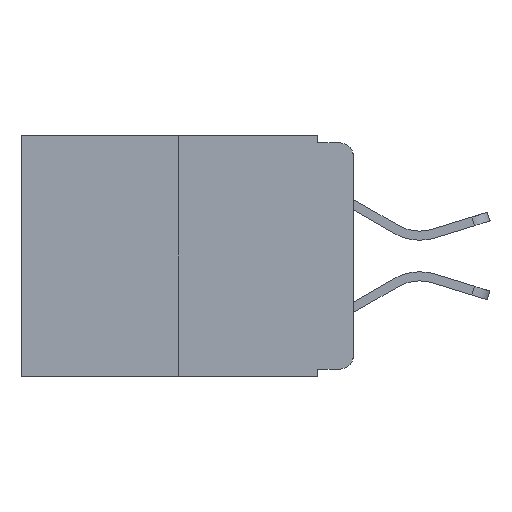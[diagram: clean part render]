
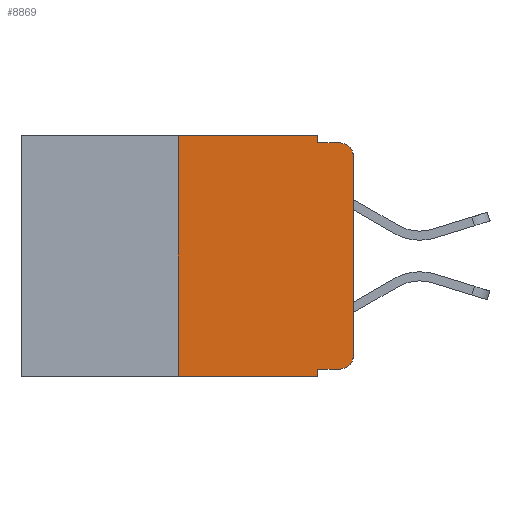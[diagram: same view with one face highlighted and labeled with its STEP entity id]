
A CAD part, left-side view. The second image highlights one B-rep face of the part: STEP entity #8869.
In plain terms, the highlighted planar face has unit normal (-1, 0, 0).
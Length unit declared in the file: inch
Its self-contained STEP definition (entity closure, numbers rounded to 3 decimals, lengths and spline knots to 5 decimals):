
#67 = ORIENTED_EDGE ( 'NONE', *, *, #6273, .F. ) ;
#86 = ORIENTED_EDGE ( 'NONE', *, *, #17245, .T. ) ;
#138 = VERTEX_POINT ( 'NONE', #15224 ) ;
#441 = CARTESIAN_POINT ( 'NONE',  ( 0., 0., -0.03 ) ) ;
#612 = EDGE_CURVE ( 'NONE', #138, #10915, #4521, .T. ) ;
#1225 = DIRECTION ( 'NONE',  ( 0., -1., 0. ) ) ;
#1445 = CARTESIAN_POINT ( 'NONE',  ( 0., 0.25, 0. ) ) ;
#1669 = DIRECTION ( 'NONE',  ( 0., -1., 0. ) ) ;
#1747 = EDGE_CURVE ( 'NONE', #2428, #138, #6983, .T. ) ;
#1871 = VECTOR ( 'NONE', #5521, 39.37008 ) ;
#2053 = DIRECTION ( 'NONE',  ( 0., 0., 1. ) ) ;
#2428 = VERTEX_POINT ( 'NONE', #8044 ) ;
#2484 = CARTESIAN_POINT ( 'NONE',  ( 0., 0.25, -0.343 ) ) ;
#2656 = CARTESIAN_POINT ( 'NONE',  ( 0., 0.473, 0. ) ) ;
#2791 = CARTESIAN_POINT ( 'NONE',  ( 0., 0.051, -0.333 ) ) ;
#2795 = EDGE_CURVE ( 'NONE', #9002, #14199, #11804, .T. ) ;
#3667 = LINE ( 'NONE', #18136, #10806 ) ;
#3687 = ORIENTED_EDGE ( 'NONE', *, *, #612, .T. ) ;
#3758 = VECTOR ( 'NONE', #16440, 39.37008 ) ;
#4008 = AXIS2_PLACEMENT_3D ( 'NONE', #2656, #12648, #4095 ) ;
#4095 = DIRECTION ( 'NONE',  ( 0., 0., -1. ) ) ;
#4148 = ORIENTED_EDGE ( 'NONE', *, *, #7474, .F. ) ;
#4521 = LINE ( 'NONE', #5185, #7886 ) ;
#5185 = CARTESIAN_POINT ( 'NONE',  ( 0., 0., 0. ) ) ;
#5221 = EDGE_CURVE ( 'NONE', #10643, #11042, #16909, .T. ) ;
#5313 = CARTESIAN_POINT ( 'NONE',  ( 0., 0.051, 0. ) ) ;
#5521 = DIRECTION ( 'NONE',  ( 0., -1., 0. ) ) ;
#5792 = LINE ( 'NONE', #8795, #12901 ) ;
#5870 = CARTESIAN_POINT ( 'NONE',  ( 0., 0.473, -0.343 ) ) ;
#6273 = EDGE_CURVE ( 'NONE', #16068, #11042, #18173, .T. ) ;
#6460 = CARTESIAN_POINT ( 'NONE',  ( 0., 0.02, -0.313 ) ) ;
#6477 = DIRECTION ( 'NONE',  ( -1., 0., 0. ) ) ;
#6510 = CARTESIAN_POINT ( 'NONE',  ( 0., 0.051, -0.343 ) ) ;
#6549 = DIRECTION ( 'NONE',  ( -1., 0., 0. ) ) ;
#6592 = DIRECTION ( 'NONE',  ( 0., 0., -1. ) ) ;
#6983 = CIRCLE ( 'NONE', #7169, 0.02 ) ;
#7169 = AXIS2_PLACEMENT_3D ( 'NONE', #6460, #6549, #6592 ) ;
#7174 = VECTOR ( 'NONE', #2053, 39.37008 ) ;
#7474 = EDGE_CURVE ( 'NONE', #10643, #9002, #14667, .T. ) ;
#7886 = VECTOR ( 'NONE', #10283, 39.37008 ) ;
#8044 = CARTESIAN_POINT ( 'NONE',  ( 0., 0.02, -0.333 ) ) ;
#8179 = CIRCLE ( 'NONE', #13635, 0.02 ) ;
#8515 = CARTESIAN_POINT ( 'NONE',  ( 0., 0.02, -0.01 ) ) ;
#8618 = ORIENTED_EDGE ( 'NONE', *, *, #2795, .F. ) ;
#8795 = CARTESIAN_POINT ( 'NONE',  ( 0., 0.051, -0.01 ) ) ;
#8826 = DIRECTION ( 'NONE',  ( 0., 0., -1. ) ) ;
#8834 = ORIENTED_EDGE ( 'NONE', *, *, #1747, .T. ) ;
#8869 = ADVANCED_FACE ( 'NONE', ( #12889 ), #11194, .F. ) ;
#9000 = CARTESIAN_POINT ( 'NONE',  ( 0., 0.051, 0. ) ) ;
#9002 = VERTEX_POINT ( 'NONE', #1445 ) ;
#9023 = DIRECTION ( 'NONE',  ( 0., 0., -1. ) ) ;
#9049 = ORIENTED_EDGE ( 'NONE', *, *, #16284, .F. ) ;
#9280 = LINE ( 'NONE', #11894, #12655 ) ;
#10164 = VERTEX_POINT ( 'NONE', #8515 ) ;
#10283 = DIRECTION ( 'NONE',  ( 0., 0., 1. ) ) ;
#10498 = EDGE_LOOP ( 'NONE', ( #3687, #13173, #17780, #9049, #8618, #4148, #11730, #67, #86, #8834 ) ) ;
#10621 = CARTESIAN_POINT ( 'NONE',  ( 0., 0.25, 0. ) ) ;
#10643 = VERTEX_POINT ( 'NONE', #2484 ) ;
#10793 = VECTOR ( 'NONE', #8826, 39.37008 ) ;
#10806 = VECTOR ( 'NONE', #1225, 39.37008 ) ;
#10915 = VERTEX_POINT ( 'NONE', #441 ) ;
#11042 = VERTEX_POINT ( 'NONE', #6510 ) ;
#11194 = PLANE ( 'NONE',  #4008 ) ;
#11730 = ORIENTED_EDGE ( 'NONE', *, *, #5221, .T. ) ;
#11804 = LINE ( 'NONE', #13671, #3758 ) ;
#11894 = CARTESIAN_POINT ( 'NONE',  ( 0., 0.051, 0. ) ) ;
#12648 = DIRECTION ( 'NONE',  ( 1., 0., 0. ) ) ;
#12655 = VECTOR ( 'NONE', #9023, 39.37008 ) ;
#12889 = FACE_OUTER_BOUND ( 'NONE', #10498, .T. ) ;
#12901 = VECTOR ( 'NONE', #1669, 39.37008 ) ;
#13173 = ORIENTED_EDGE ( 'NONE', *, *, #17015, .T. ) ;
#13635 = AXIS2_PLACEMENT_3D ( 'NONE', #14926, #6477, #16289 ) ;
#13671 = CARTESIAN_POINT ( 'NONE',  ( 0., 0.473, 0. ) ) ;
#14199 = VERTEX_POINT ( 'NONE', #9000 ) ;
#14667 = LINE ( 'NONE', #10621, #7174 ) ;
#14926 = CARTESIAN_POINT ( 'NONE',  ( 0., 0.02, -0.03 ) ) ;
#15224 = CARTESIAN_POINT ( 'NONE',  ( 0., 0., -0.313 ) ) ;
#15605 = EDGE_CURVE ( 'NONE', #15954, #10164, #5792, .T. ) ;
#15954 = VERTEX_POINT ( 'NONE', #17818 ) ;
#16068 = VERTEX_POINT ( 'NONE', #2791 ) ;
#16284 = EDGE_CURVE ( 'NONE', #14199, #15954, #9280, .T. ) ;
#16289 = DIRECTION ( 'NONE',  ( 0., 0., -1. ) ) ;
#16440 = DIRECTION ( 'NONE',  ( 0., -1., 0. ) ) ;
#16909 = LINE ( 'NONE', #5870, #1871 ) ;
#17015 = EDGE_CURVE ( 'NONE', #10915, #10164, #8179, .T. ) ;
#17245 = EDGE_CURVE ( 'NONE', #16068, #2428, #3667, .T. ) ;
#17780 = ORIENTED_EDGE ( 'NONE', *, *, #15605, .F. ) ;
#17818 = CARTESIAN_POINT ( 'NONE',  ( 0., 0.051, -0.01 ) ) ;
#18136 = CARTESIAN_POINT ( 'NONE',  ( 0., 0.051, -0.333 ) ) ;
#18173 = LINE ( 'NONE', #5313, #10793 ) ;
